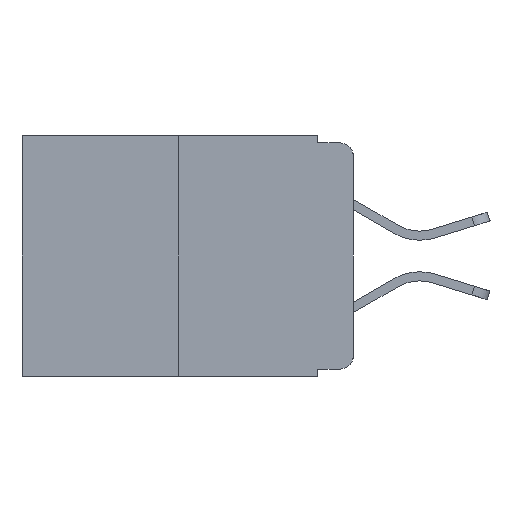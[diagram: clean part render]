
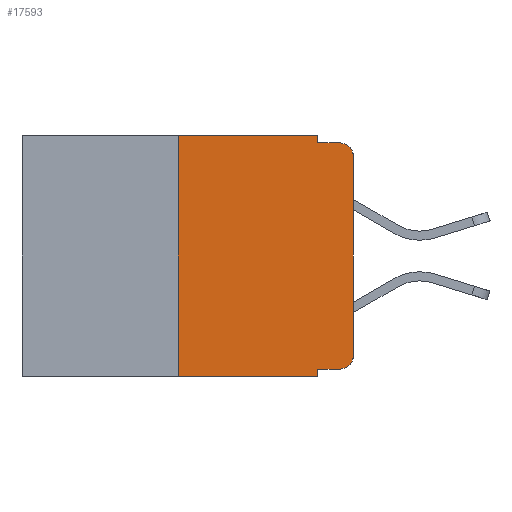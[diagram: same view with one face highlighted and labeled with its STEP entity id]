
A CAD part, left-side view. The second image highlights one B-rep face of the part: STEP entity #17593.
In plain terms, the highlighted planar face has unit normal (-1, 0, 0).
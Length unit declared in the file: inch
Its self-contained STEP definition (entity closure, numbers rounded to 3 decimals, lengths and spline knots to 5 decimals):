
#109 = EDGE_CURVE ( 'NONE', #13373, #5450, #7792, .T. ) ;
#408 = VERTEX_POINT ( 'NONE', #21440 ) ;
#694 = DIRECTION ( 'NONE',  ( -1., 0., 0. ) ) ;
#1112 = CARTESIAN_POINT ( 'NONE',  ( 0., 0.473, 0. ) ) ;
#1173 = ORIENTED_EDGE ( 'NONE', *, *, #21019, .F. ) ;
#1180 = CARTESIAN_POINT ( 'NONE',  ( 0., 0.051, -0.333 ) ) ;
#1304 = VECTOR ( 'NONE', #4312, 39.37008 ) ;
#1551 = DIRECTION ( 'NONE',  ( -1., 0., 0. ) ) ;
#1599 = VERTEX_POINT ( 'NONE', #5226 ) ;
#1864 = LINE ( 'NONE', #22993, #16827 ) ;
#2272 = ORIENTED_EDGE ( 'NONE', *, *, #19830, .F. ) ;
#2341 = VECTOR ( 'NONE', #7924, 39.37008 ) ;
#3419 = DIRECTION ( 'NONE',  ( 0., 0., -1. ) ) ;
#3774 = CIRCLE ( 'NONE', #11262, 0.02 ) ;
#4007 = VECTOR ( 'NONE', #22067, 39.37008 ) ;
#4111 = EDGE_CURVE ( 'NONE', #408, #19016, #1864, .T. ) ;
#4168 = CARTESIAN_POINT ( 'NONE',  ( 0., 0.473, -0.343 ) ) ;
#4312 = DIRECTION ( 'NONE',  ( 0., 0., 1. ) ) ;
#4412 = CARTESIAN_POINT ( 'NONE',  ( 0., 0.25, 0. ) ) ;
#4424 = DIRECTION ( 'NONE',  ( 0., 0., -1. ) ) ;
#4783 = EDGE_CURVE ( 'NONE', #19016, #12010, #14015, .T. ) ;
#5226 = CARTESIAN_POINT ( 'NONE',  ( 0., 0.051, -0.343 ) ) ;
#5450 = VERTEX_POINT ( 'NONE', #19208 ) ;
#5886 = CARTESIAN_POINT ( 'NONE',  ( 0., 0.051, -0.01 ) ) ;
#6451 = ORIENTED_EDGE ( 'NONE', *, *, #4783, .T. ) ;
#6606 = EDGE_CURVE ( 'NONE', #23721, #10104, #22415, .T. ) ;
#7792 = LINE ( 'NONE', #13674, #2341 ) ;
#7924 = DIRECTION ( 'NONE',  ( 0., -1., 0. ) ) ;
#8220 = CARTESIAN_POINT ( 'NONE',  ( 0., 0.051, 0. ) ) ;
#8326 = EDGE_CURVE ( 'NONE', #5450, #408, #3774, .T. ) ;
#8968 = ORIENTED_EDGE ( 'NONE', *, *, #18553, .F. ) ;
#9570 = DIRECTION ( 'NONE',  ( 0., 0., 1. ) ) ;
#10104 = VERTEX_POINT ( 'NONE', #22813 ) ;
#10178 = ORIENTED_EDGE ( 'NONE', *, *, #6606, .F. ) ;
#10354 = AXIS2_PLACEMENT_3D ( 'NONE', #13396, #1551, #3419 ) ;
#11262 = AXIS2_PLACEMENT_3D ( 'NONE', #22198, #694, #22459 ) ;
#11849 = ORIENTED_EDGE ( 'NONE', *, *, #4111, .T. ) ;
#11865 = CARTESIAN_POINT ( 'NONE',  ( 0., 0.051, 0. ) ) ;
#11899 = CARTESIAN_POINT ( 'NONE',  ( 0., 0.051, -0.01 ) ) ;
#12010 = VERTEX_POINT ( 'NONE', #17349 ) ;
#12430 = VERTEX_POINT ( 'NONE', #11899 ) ;
#12483 = PLANE ( 'NONE',  #13104 ) ;
#13056 = EDGE_CURVE ( 'NONE', #10104, #12430, #20576, .T. ) ;
#13104 = AXIS2_PLACEMENT_3D ( 'NONE', #14623, #16176, #4424 ) ;
#13373 = VERTEX_POINT ( 'NONE', #1180 ) ;
#13396 = CARTESIAN_POINT ( 'NONE',  ( 0., 0.02, -0.03 ) ) ;
#13439 = ORIENTED_EDGE ( 'NONE', *, *, #23541, .T. ) ;
#13674 = CARTESIAN_POINT ( 'NONE',  ( 0., 0.051, -0.333 ) ) ;
#13811 = LINE ( 'NONE', #20001, #1304 ) ;
#14015 = CIRCLE ( 'NONE', #10354, 0.02 ) ;
#14316 = EDGE_LOOP ( 'NONE', ( #11849, #6451, #8968, #22238, #10178, #1173, #13439, #2272, #14423, #18649 ) ) ;
#14423 = ORIENTED_EDGE ( 'NONE', *, *, #109, .T. ) ;
#14623 = CARTESIAN_POINT ( 'NONE',  ( 0., 0.473, 0. ) ) ;
#14918 = VECTOR ( 'NONE', #19606, 39.37008 ) ;
#15834 = DIRECTION ( 'NONE',  ( 0., -1., 0. ) ) ;
#15899 = CARTESIAN_POINT ( 'NONE',  ( 0., 0.25, -0.343 ) ) ;
#16099 = VERTEX_POINT ( 'NONE', #15899 ) ;
#16176 = DIRECTION ( 'NONE',  ( 1., 0., 0. ) ) ;
#16827 = VECTOR ( 'NONE', #9570, 39.37008 ) ;
#17349 = CARTESIAN_POINT ( 'NONE',  ( 0., 0.02, -0.01 ) ) ;
#17572 = CARTESIAN_POINT ( 'NONE',  ( 0., 0., -0.03 ) ) ;
#17593 = ADVANCED_FACE ( 'NONE', ( #19337 ), #12483, .F. ) ;
#18553 = EDGE_CURVE ( 'NONE', #12430, #12010, #20184, .T. ) ;
#18649 = ORIENTED_EDGE ( 'NONE', *, *, #8326, .T. ) ;
#19016 = VERTEX_POINT ( 'NONE', #17572 ) ;
#19208 = CARTESIAN_POINT ( 'NONE',  ( 0., 0.02, -0.333 ) ) ;
#19337 = FACE_OUTER_BOUND ( 'NONE', #14316, .T. ) ;
#19606 = DIRECTION ( 'NONE',  ( 0., -1., 0. ) ) ;
#19668 = DIRECTION ( 'NONE',  ( 0., 0., -1. ) ) ;
#19830 = EDGE_CURVE ( 'NONE', #13373, #1599, #22886, .T. ) ;
#20001 = CARTESIAN_POINT ( 'NONE',  ( 0., 0.25, 0. ) ) ;
#20184 = LINE ( 'NONE', #5886, #22901 ) ;
#20342 = DIRECTION ( 'NONE',  ( 0., -1., 0. ) ) ;
#20576 = LINE ( 'NONE', #11865, #23877 ) ;
#20921 = VECTOR ( 'NONE', #20342, 39.37008 ) ;
#21019 = EDGE_CURVE ( 'NONE', #16099, #23721, #13811, .T. ) ;
#21440 = CARTESIAN_POINT ( 'NONE',  ( 0., 0., -0.313 ) ) ;
#22067 = DIRECTION ( 'NONE',  ( 0., 0., -1. ) ) ;
#22198 = CARTESIAN_POINT ( 'NONE',  ( 0., 0.02, -0.313 ) ) ;
#22238 = ORIENTED_EDGE ( 'NONE', *, *, #13056, .F. ) ;
#22415 = LINE ( 'NONE', #1112, #20921 ) ;
#22459 = DIRECTION ( 'NONE',  ( 0., 0., -1. ) ) ;
#22813 = CARTESIAN_POINT ( 'NONE',  ( 0., 0.051, 0. ) ) ;
#22886 = LINE ( 'NONE', #8220, #4007 ) ;
#22901 = VECTOR ( 'NONE', #15834, 39.37008 ) ;
#22993 = CARTESIAN_POINT ( 'NONE',  ( 0., 0., 0. ) ) ;
#23087 = LINE ( 'NONE', #4168, #14918 ) ;
#23541 = EDGE_CURVE ( 'NONE', #16099, #1599, #23087, .T. ) ;
#23721 = VERTEX_POINT ( 'NONE', #4412 ) ;
#23877 = VECTOR ( 'NONE', #19668, 39.37008 ) ;
